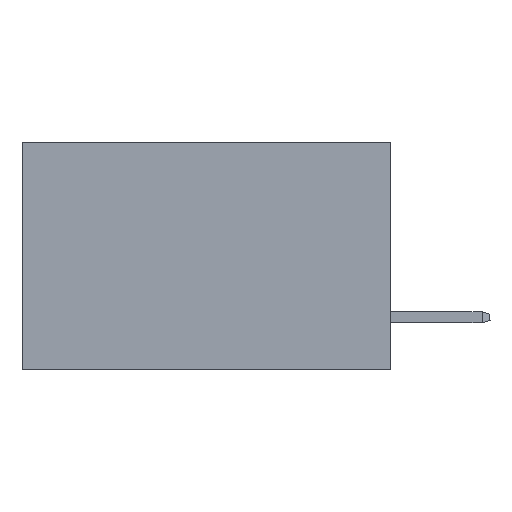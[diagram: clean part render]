
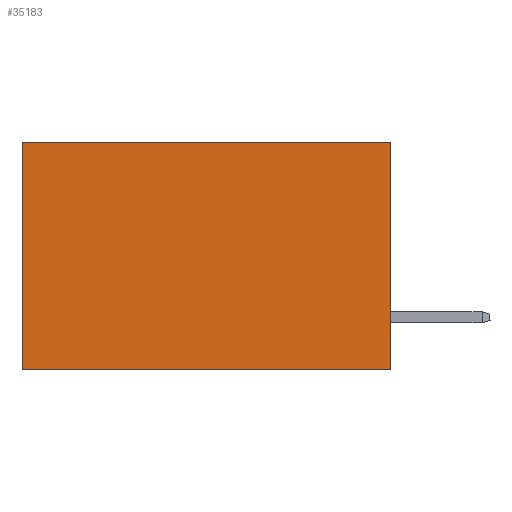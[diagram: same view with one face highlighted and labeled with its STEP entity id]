
A CAD part, left-side view. The second image highlights one B-rep face of the part: STEP entity #35183.
In plain terms, the highlighted planar face has unit normal (-1, 0, 0).
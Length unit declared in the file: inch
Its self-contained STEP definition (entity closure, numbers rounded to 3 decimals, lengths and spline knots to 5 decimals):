
#1704 = ORIENTED_EDGE ( 'NONE', *, *, #7931, .T. ) ;
#6376 = EDGE_CURVE ( 'NONE', #8310, #16729, #26195, .T. ) ;
#7931 = EDGE_CURVE ( 'NONE', #25060, #22906, #26429, .T. ) ;
#8136 = AXIS2_PLACEMENT_3D ( 'NONE', #17754, #44451, #40853 ) ;
#8310 = VERTEX_POINT ( 'NONE', #9035 ) ;
#9035 = CARTESIAN_POINT ( 'NONE',  ( 0.2875, 0., 0. ) ) ;
#9057 = DIRECTION ( 'NONE',  ( 0., 1., 0. ) ) ;
#9337 = CARTESIAN_POINT ( 'NONE',  ( 0.2875, 0., -0.37 ) ) ;
#10801 = CARTESIAN_POINT ( 'NONE',  ( 0.2875, 0.6, 0. ) ) ;
#12098 = CARTESIAN_POINT ( 'NONE',  ( 0.2875, 0., 0. ) ) ;
#12303 = ORIENTED_EDGE ( 'NONE', *, *, #6376, .F. ) ;
#15013 = EDGE_LOOP ( 'NONE', ( #1704, #29254, #12303, #19585 ) ) ;
#16376 = VECTOR ( 'NONE', #30985, 39.37008 ) ;
#16729 = VERTEX_POINT ( 'NONE', #9337 ) ;
#17166 = CARTESIAN_POINT ( 'NONE',  ( 0.2875, 0., -0.37 ) ) ;
#17754 = CARTESIAN_POINT ( 'NONE',  ( 0.2875, 0., 0. ) ) ;
#19585 = ORIENTED_EDGE ( 'NONE', *, *, #42956, .T. ) ;
#22906 = VERTEX_POINT ( 'NONE', #33517 ) ;
#24760 = DIRECTION ( 'NONE',  ( 0., 0., -1. ) ) ;
#25060 = VERTEX_POINT ( 'NONE', #10801 ) ;
#26195 = LINE ( 'NONE', #12098, #16376 ) ;
#26429 = LINE ( 'NONE', #43732, #29402 ) ;
#26886 = FACE_OUTER_BOUND ( 'NONE', #15013, .T. ) ;
#27563 = VECTOR ( 'NONE', #31873, 39.37008 ) ;
#28929 = CARTESIAN_POINT ( 'NONE',  ( 0.2875, 0., 0. ) ) ;
#29254 = ORIENTED_EDGE ( 'NONE', *, *, #30896, .F. ) ;
#29402 = VECTOR ( 'NONE', #24760, 39.37008 ) ;
#30124 = VECTOR ( 'NONE', #9057, 39.37008 ) ;
#30896 = EDGE_CURVE ( 'NONE', #16729, #22906, #43701, .T. ) ;
#30985 = DIRECTION ( 'NONE',  ( 0., 0., -1. ) ) ;
#31873 = DIRECTION ( 'NONE',  ( 0., 1., 0. ) ) ;
#33517 = CARTESIAN_POINT ( 'NONE',  ( 0.2875, 0.6, -0.37 ) ) ;
#35183 = ADVANCED_FACE ( 'NONE', ( #26886 ), #36824, .F. ) ;
#36824 = PLANE ( 'NONE',  #8136 ) ;
#40853 = DIRECTION ( 'NONE',  ( 0., 0., -1. ) ) ;
#41905 = LINE ( 'NONE', #28929, #27563 ) ;
#42956 = EDGE_CURVE ( 'NONE', #8310, #25060, #41905, .T. ) ;
#43701 = LINE ( 'NONE', #17166, #30124 ) ;
#43732 = CARTESIAN_POINT ( 'NONE',  ( 0.2875, 0.6, 0. ) ) ;
#44451 = DIRECTION ( 'NONE',  ( 1., 0., 0. ) ) ;
